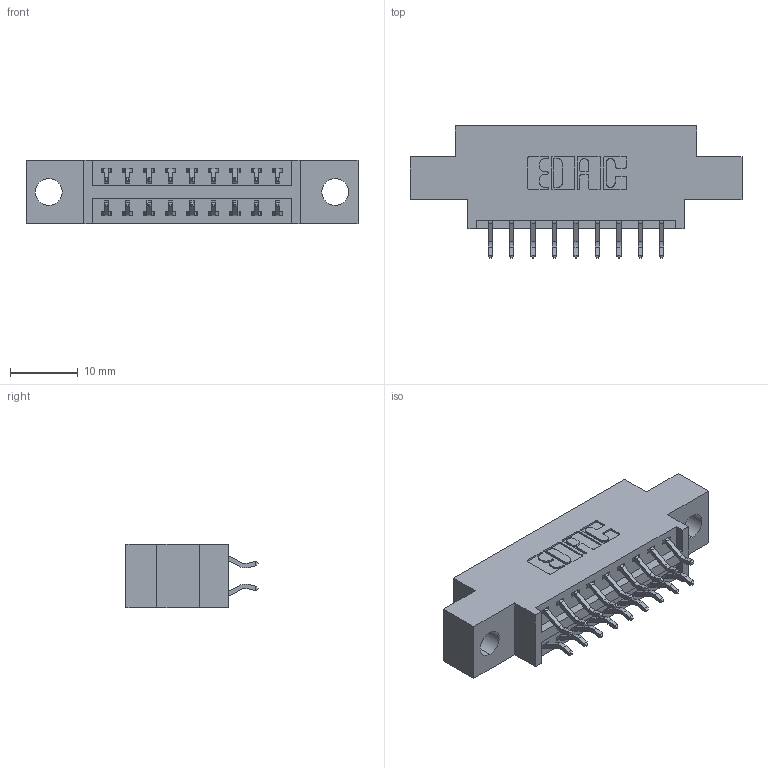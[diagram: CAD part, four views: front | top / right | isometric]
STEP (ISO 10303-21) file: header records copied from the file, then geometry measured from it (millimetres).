
FILE_DESCRIPTION (( 'STEP AP203' ), '1' );
FILE_NAME ('396-018-556-804.STEP', '2019-11-01T17:58:13', ( '' ), ( '' ), 'SwSTEP 2.0', 'SolidWorks 2016', '' );
FILE_SCHEMA (( 'CONFIG_CONTROL_DESIGN' ));
Length unit declared in the file: inch
Products named in the file (3): 346 Part_0.170 Offset - 0.156 Dia-TH; 345-292-001_556 Tail; 396-018-556-804
Assembly tree (19 placements, depth 2):
  396-018-556-804
    346 Part_0.170 Offset - 0.156 Dia-TH
    345-292-001_556 Tail  x18
Bounding box: 49.15 x 19.57 x 9.4 mm (x, y, z)
Volume: 4293.2 mm3; surface area: 5358.8 mm2
Topology: 19 solids, 19 shells, 1170 faces, 3455 edges, 2278 vertices
Faces by surface type: plane 782, cylinder 388
Entity records: 10671 total; most frequent: CARTESIAN_POINT 1820, ORIENTED_EDGE 1742, DIRECTION 1643, EDGE_CURVE 871, LINE 695, VECTOR 695, VERTEX_POINT 578, AXIS2_PLACEMENT_3D 474
